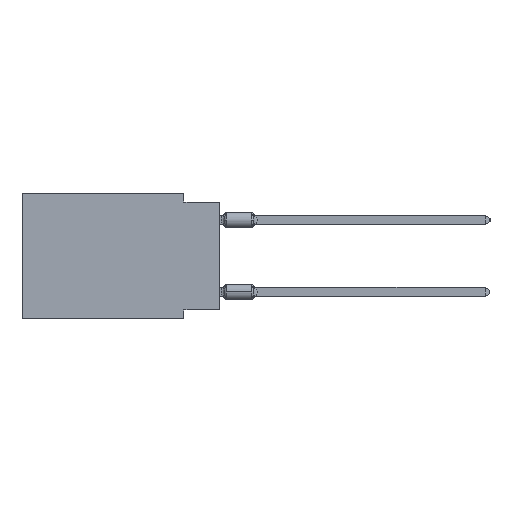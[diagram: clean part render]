
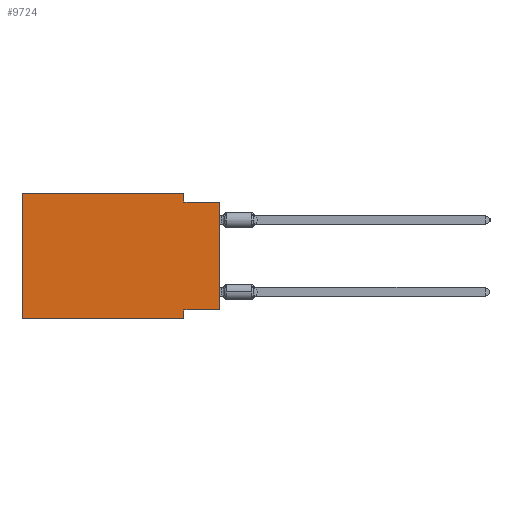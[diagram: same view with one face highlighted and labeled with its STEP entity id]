
A CAD part, left-side view. The second image highlights one B-rep face of the part: STEP entity #9724.
In plain terms, the highlighted planar face has unit normal (-1, 0, 0).
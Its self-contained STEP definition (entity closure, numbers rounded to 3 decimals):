
#380 = VECTOR ( 'NONE', #7827, 1000. ) ;
#1146 = CARTESIAN_POINT ( 'NONE',  ( 0., 13.97, -8.89 ) ) ;
#1300 = VERTEX_POINT ( 'NONE', #19811 ) ;
#1443 = VECTOR ( 'NONE', #11839, 1000. ) ;
#2222 = ORIENTED_EDGE ( 'NONE', *, *, #19993, .F. ) ;
#2303 = LINE ( 'NONE', #13083, #380 ) ;
#2759 = DIRECTION ( 'NONE',  ( 0., 0., 1. ) ) ;
#2840 = LINE ( 'NONE', #17705, #17502 ) ;
#3246 = ORIENTED_EDGE ( 'NONE', *, *, #19202, .F. ) ;
#3900 = VECTOR ( 'NONE', #16898, 1000. ) ;
#4248 = VERTEX_POINT ( 'NONE', #4848 ) ;
#4429 = CARTESIAN_POINT ( 'NONE',  ( 0., 0., -8.255 ) ) ;
#4848 = CARTESIAN_POINT ( 'NONE',  ( 0., 2.54, 0. ) ) ;
#5338 = CARTESIAN_POINT ( 'NONE',  ( 0., 2.54, -8.255 ) ) ;
#5380 = DIRECTION ( 'NONE',  ( 0., 0., -1. ) ) ;
#5513 = CARTESIAN_POINT ( 'NONE',  ( 0., 0., 0. ) ) ;
#5768 = VECTOR ( 'NONE', #5380, 1000. ) ;
#6183 = EDGE_CURVE ( 'NONE', #21962, #23077, #2840, .T. ) ;
#7642 = VECTOR ( 'NONE', #2759, 1000. ) ;
#7827 = DIRECTION ( 'NONE',  ( 0., 0., -1. ) ) ;
#7991 = LINE ( 'NONE', #4429, #23754 ) ;
#8748 = CARTESIAN_POINT ( 'NONE',  ( 0., 2.54, -8.89 ) ) ;
#9392 = LINE ( 'NONE', #18494, #3900 ) ;
#9472 = EDGE_CURVE ( 'NONE', #16742, #24060, #9392, .T. ) ;
#9724 = ADVANCED_FACE ( 'NONE', ( #23348 ), #16089, .F. ) ;
#10233 = CARTESIAN_POINT ( 'NONE',  ( 0., 13.97, 0. ) ) ;
#10241 = ORIENTED_EDGE ( 'NONE', *, *, #23650, .T. ) ;
#11518 = LINE ( 'NONE', #5513, #11633 ) ;
#11597 = LINE ( 'NONE', #18876, #1443 ) ;
#11633 = VECTOR ( 'NONE', #12997, 1000. ) ;
#11740 = EDGE_CURVE ( 'NONE', #4248, #16742, #2303, .T. ) ;
#11839 = DIRECTION ( 'NONE',  ( 0., -1., 0. ) ) ;
#11903 = DIRECTION ( 'NONE',  ( 1., 0., 0. ) ) ;
#11984 = ORIENTED_EDGE ( 'NONE', *, *, #6183, .T. ) ;
#12997 = DIRECTION ( 'NONE',  ( 0., 0., 1. ) ) ;
#13083 = CARTESIAN_POINT ( 'NONE',  ( 0., 2.54, 0. ) ) ;
#13166 = VERTEX_POINT ( 'NONE', #5338 ) ;
#14233 = ORIENTED_EDGE ( 'NONE', *, *, #20805, .F. ) ;
#14815 = CARTESIAN_POINT ( 'NONE',  ( 0., 0., -0.635 ) ) ;
#15851 = ORIENTED_EDGE ( 'NONE', *, *, #9472, .F. ) ;
#16040 = AXIS2_PLACEMENT_3D ( 'NONE', #17579, #11903, #23233 ) ;
#16089 = PLANE ( 'NONE',  #16040 ) ;
#16556 = LINE ( 'NONE', #24050, #5768 ) ;
#16742 = VERTEX_POINT ( 'NONE', #20306 ) ;
#16898 = DIRECTION ( 'NONE',  ( 0., -1., 0. ) ) ;
#17502 = VECTOR ( 'NONE', #23839, 1000. ) ;
#17579 = CARTESIAN_POINT ( 'NONE',  ( 0., 13.97, 0. ) ) ;
#17705 = CARTESIAN_POINT ( 'NONE',  ( 0., 13.97, -8.89 ) ) ;
#18494 = CARTESIAN_POINT ( 'NONE',  ( 0., 0., -0.635 ) ) ;
#18656 = CARTESIAN_POINT ( 'NONE',  ( 0., 13.97, 0. ) ) ;
#18876 = CARTESIAN_POINT ( 'NONE',  ( 0., 13.97, 0. ) ) ;
#19202 = EDGE_CURVE ( 'NONE', #21962, #22419, #23279, .T. ) ;
#19405 = DIRECTION ( 'NONE',  ( 0., 1., 0. ) ) ;
#19811 = CARTESIAN_POINT ( 'NONE',  ( 0., 0., -8.255 ) ) ;
#19993 = EDGE_CURVE ( 'NONE', #1300, #13166, #7991, .T. ) ;
#20126 = EDGE_LOOP ( 'NONE', ( #10241, #15851, #21856, #14233, #3246, #11984, #24124, #2222 ) ) ;
#20306 = CARTESIAN_POINT ( 'NONE',  ( 0., 2.54, -0.635 ) ) ;
#20805 = EDGE_CURVE ( 'NONE', #22419, #4248, #11597, .T. ) ;
#21250 = EDGE_CURVE ( 'NONE', #13166, #23077, #16556, .T. ) ;
#21856 = ORIENTED_EDGE ( 'NONE', *, *, #11740, .F. ) ;
#21962 = VERTEX_POINT ( 'NONE', #1146 ) ;
#22419 = VERTEX_POINT ( 'NONE', #18656 ) ;
#23077 = VERTEX_POINT ( 'NONE', #8748 ) ;
#23233 = DIRECTION ( 'NONE',  ( 0., 0., -1. ) ) ;
#23279 = LINE ( 'NONE', #10233, #7642 ) ;
#23348 = FACE_OUTER_BOUND ( 'NONE', #20126, .T. ) ;
#23650 = EDGE_CURVE ( 'NONE', #1300, #24060, #11518, .T. ) ;
#23754 = VECTOR ( 'NONE', #19405, 1000. ) ;
#23839 = DIRECTION ( 'NONE',  ( 0., -1., 0. ) ) ;
#24050 = CARTESIAN_POINT ( 'NONE',  ( 0., 2.54, -8.89 ) ) ;
#24060 = VERTEX_POINT ( 'NONE', #14815 ) ;
#24124 = ORIENTED_EDGE ( 'NONE', *, *, #21250, .F. ) ;
